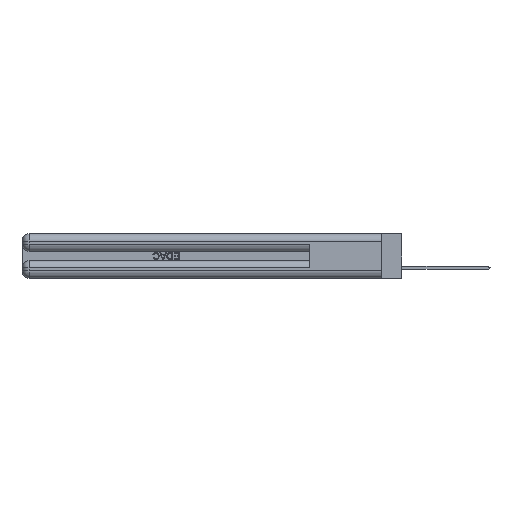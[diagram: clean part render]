
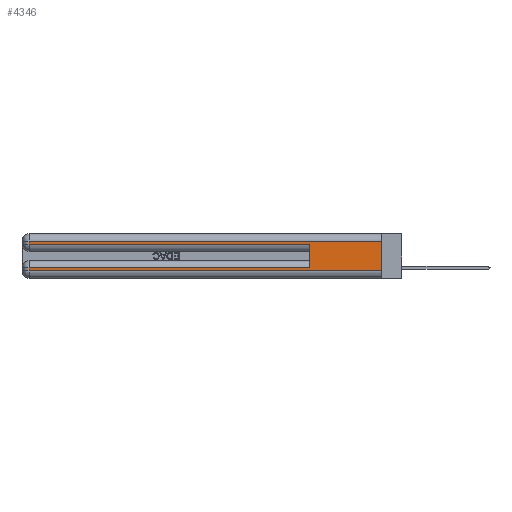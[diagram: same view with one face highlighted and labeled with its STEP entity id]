
A CAD part, left-side view. The second image highlights one B-rep face of the part: STEP entity #4346.
In plain terms, the highlighted planar face has unit normal (-1, 0, 0).
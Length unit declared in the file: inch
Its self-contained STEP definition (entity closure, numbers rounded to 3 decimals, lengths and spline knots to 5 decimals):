
#128 = LINE ( 'NONE', #36368, #4885 ) ;
#257 = ORIENTED_EDGE ( 'NONE', *, *, #23748, .T. ) ;
#785 = VECTOR ( 'NONE', #31219, 39.37008 ) ;
#831 = CARTESIAN_POINT ( 'NONE',  ( 0., 0., 0.31 ) ) ;
#1458 = DIRECTION ( 'NONE',  ( 0., -1., 0. ) ) ;
#2643 = DIRECTION ( 'NONE',  ( 1., 0., 0. ) ) ;
#2883 = VECTOR ( 'NONE', #10239, 39.37008 ) ;
#3351 = ORIENTED_EDGE ( 'NONE', *, *, #7636, .T. ) ;
#3577 = VECTOR ( 'NONE', #20457, 39.37008 ) ;
#4346 = ADVANCED_FACE ( 'NONE', ( #32133 ), #15222, .F. ) ;
#4885 = VECTOR ( 'NONE', #12935, 39.37008 ) ;
#5052 = CARTESIAN_POINT ( 'NONE',  ( 0., 0., 0.06 ) ) ;
#5752 = CARTESIAN_POINT ( 'NONE',  ( 0., 2.94, 0.31 ) ) ;
#6567 = VERTEX_POINT ( 'NONE', #5752 ) ;
#6687 = CARTESIAN_POINT ( 'NONE',  ( 0., 2.94, 0.37 ) ) ;
#7132 = EDGE_LOOP ( 'NONE', ( #14302, #24974, #3351, #22803, #27662, #20968, #30513, #257 ) ) ;
#7636 = EDGE_CURVE ( 'NONE', #6567, #13436, #37647, .T. ) ;
#7788 = VECTOR ( 'NONE', #25417, 39.37008 ) ;
#9277 = CARTESIAN_POINT ( 'NONE',  ( 0., 2.94, 0.06 ) ) ;
#9323 = LINE ( 'NONE', #11636, #35476 ) ;
#9948 = VERTEX_POINT ( 'NONE', #38171 ) ;
#10057 = LINE ( 'NONE', #28313, #31914 ) ;
#10239 = DIRECTION ( 'NONE',  ( 0., 0., -1. ) ) ;
#10852 = VERTEX_POINT ( 'NONE', #29520 ) ;
#10914 = AXIS2_PLACEMENT_3D ( 'NONE', #16262, #2643, #22771 ) ;
#11636 = CARTESIAN_POINT ( 'NONE',  ( 0., 0., 0.285 ) ) ;
#12935 = DIRECTION ( 'NONE',  ( 0., -1., 0. ) ) ;
#13385 = CARTESIAN_POINT ( 'NONE',  ( 0., 0.6, 0.085 ) ) ;
#13436 = VERTEX_POINT ( 'NONE', #42351 ) ;
#14302 = ORIENTED_EDGE ( 'NONE', *, *, #25611, .F. ) ;
#15222 = PLANE ( 'NONE',  #10914 ) ;
#16262 = CARTESIAN_POINT ( 'NONE',  ( 0., 0., 0.37 ) ) ;
#17498 = CARTESIAN_POINT ( 'NONE',  ( 0., 0.6, 0.145 ) ) ;
#18990 = LINE ( 'NONE', #31367, #785 ) ;
#20457 = DIRECTION ( 'NONE',  ( 0., 0., 1. ) ) ;
#20968 = ORIENTED_EDGE ( 'NONE', *, *, #34050, .T. ) ;
#22771 = DIRECTION ( 'NONE',  ( 0., 0., -1. ) ) ;
#22803 = ORIENTED_EDGE ( 'NONE', *, *, #28379, .T. ) ;
#23748 = EDGE_CURVE ( 'NONE', #43604, #39925, #128, .T. ) ;
#24575 = DIRECTION ( 'NONE',  ( 0., 0., -1. ) ) ;
#24719 = DIRECTION ( 'NONE',  ( 0., 1., 0. ) ) ;
#24974 = ORIENTED_EDGE ( 'NONE', *, *, #42189, .T. ) ;
#25417 = DIRECTION ( 'NONE',  ( 0., 0., -1. ) ) ;
#25611 = EDGE_CURVE ( 'NONE', #10852, #39925, #10057, .T. ) ;
#27662 = ORIENTED_EDGE ( 'NONE', *, *, #39137, .F. ) ;
#28313 = CARTESIAN_POINT ( 'NONE',  ( 0., 0., 0.37 ) ) ;
#28379 = EDGE_CURVE ( 'NONE', #13436, #37674, #9323, .T. ) ;
#29520 = CARTESIAN_POINT ( 'NONE',  ( 0., 0., 0.31 ) ) ;
#30513 = ORIENTED_EDGE ( 'NONE', *, *, #40598, .T. ) ;
#31219 = DIRECTION ( 'NONE',  ( 0., 1., 0. ) ) ;
#31367 = CARTESIAN_POINT ( 'NONE',  ( 0., 0., 0.085 ) ) ;
#31620 = LINE ( 'NONE', #831, #40268 ) ;
#31914 = VECTOR ( 'NONE', #24575, 39.37008 ) ;
#32133 = FACE_OUTER_BOUND ( 'NONE', #7132, .T. ) ;
#34050 = EDGE_CURVE ( 'NONE', #43113, #9948, #18990, .T. ) ;
#34987 = LINE ( 'NONE', #43092, #7788 ) ;
#35476 = VECTOR ( 'NONE', #1458, 39.37008 ) ;
#36368 = CARTESIAN_POINT ( 'NONE',  ( 0., 0., 0.06 ) ) ;
#37647 = LINE ( 'NONE', #6687, #2883 ) ;
#37674 = VERTEX_POINT ( 'NONE', #39399 ) ;
#38171 = CARTESIAN_POINT ( 'NONE',  ( 0., 2.94, 0.085 ) ) ;
#39137 = EDGE_CURVE ( 'NONE', #43113, #37674, #42066, .T. ) ;
#39399 = CARTESIAN_POINT ( 'NONE',  ( 0., 0.6, 0.285 ) ) ;
#39925 = VERTEX_POINT ( 'NONE', #5052 ) ;
#40268 = VECTOR ( 'NONE', #24719, 39.37008 ) ;
#40598 = EDGE_CURVE ( 'NONE', #9948, #43604, #34987, .T. ) ;
#42066 = LINE ( 'NONE', #17498, #3577 ) ;
#42189 = EDGE_CURVE ( 'NONE', #10852, #6567, #31620, .T. ) ;
#42351 = CARTESIAN_POINT ( 'NONE',  ( 0., 2.94, 0.285 ) ) ;
#43092 = CARTESIAN_POINT ( 'NONE',  ( 0., 2.94, 0.37 ) ) ;
#43113 = VERTEX_POINT ( 'NONE', #13385 ) ;
#43604 = VERTEX_POINT ( 'NONE', #9277 ) ;
